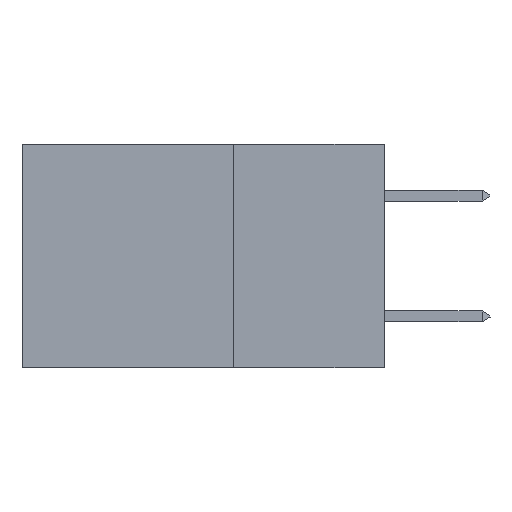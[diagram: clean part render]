
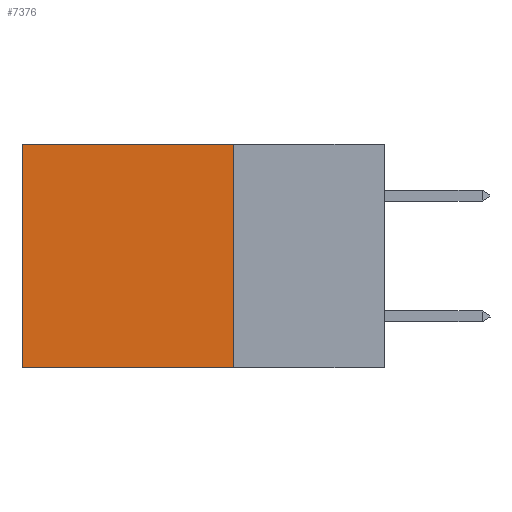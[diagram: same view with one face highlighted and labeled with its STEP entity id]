
A CAD part, left-side view. The second image highlights one B-rep face of the part: STEP entity #7376.
In plain terms, the highlighted planar face has unit normal (-1, 0, 0).
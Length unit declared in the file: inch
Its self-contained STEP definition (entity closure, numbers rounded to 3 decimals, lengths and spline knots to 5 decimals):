
#313 = CARTESIAN_POINT ( 'NONE',  ( 0.2875, 0.25, 0. ) ) ;
#563 = VECTOR ( 'NONE', #5628, 39.37008 ) ;
#585 = DIRECTION ( 'NONE',  ( 0., 0., -1. ) ) ;
#672 = CARTESIAN_POINT ( 'NONE',  ( 0.2875, 0.25, 0. ) ) ;
#883 = LINE ( 'NONE', #8996, #7415 ) ;
#1250 = DIRECTION ( 'NONE',  ( 0., 0., -1. ) ) ;
#1438 = FACE_OUTER_BOUND ( 'NONE', #3929, .T. ) ;
#1440 = DIRECTION ( 'NONE',  ( 1., 0., 0. ) ) ;
#1986 = LINE ( 'NONE', #8472, #563 ) ;
#2133 = ORIENTED_EDGE ( 'NONE', *, *, #6322, .F. ) ;
#2152 = CARTESIAN_POINT ( 'NONE',  ( 0.2875, 0.25, 0. ) ) ;
#2187 = PLANE ( 'NONE',  #6969 ) ;
#3240 = VERTEX_POINT ( 'NONE', #6380 ) ;
#3360 = VECTOR ( 'NONE', #7100, 39.37008 ) ;
#3609 = VERTEX_POINT ( 'NONE', #5166 ) ;
#3929 = EDGE_LOOP ( 'NONE', ( #6810, #2133, #7901, #4018 ) ) ;
#4018 = ORIENTED_EDGE ( 'NONE', *, *, #7542, .T. ) ;
#4304 = CARTESIAN_POINT ( 'NONE',  ( 0.2875, 0.25, 0. ) ) ;
#4471 = CARTESIAN_POINT ( 'NONE',  ( 0.2875, 0.6, 0. ) ) ;
#4871 = DIRECTION ( 'NONE',  ( 0., 0., -1. ) ) ;
#4913 = LINE ( 'NONE', #672, #5218 ) ;
#5166 = CARTESIAN_POINT ( 'NONE',  ( 0.2875, 0.6, -0.37 ) ) ;
#5218 = VECTOR ( 'NONE', #585, 39.37008 ) ;
#5628 = DIRECTION ( 'NONE',  ( 0., 1., 0. ) ) ;
#6322 = EDGE_CURVE ( 'NONE', #3240, #3609, #1986, .T. ) ;
#6380 = CARTESIAN_POINT ( 'NONE',  ( 0.2875, 0.25, -0.37 ) ) ;
#6810 = ORIENTED_EDGE ( 'NONE', *, *, #7013, .T. ) ;
#6969 = AXIS2_PLACEMENT_3D ( 'NONE', #2152, #1440, #4871 ) ;
#7013 = EDGE_CURVE ( 'NONE', #7145, #3609, #883, .T. ) ;
#7100 = DIRECTION ( 'NONE',  ( 0., 1., 0. ) ) ;
#7145 = VERTEX_POINT ( 'NONE', #4471 ) ;
#7210 = EDGE_CURVE ( 'NONE', #8713, #3240, #4913, .T. ) ;
#7376 = ADVANCED_FACE ( 'NONE', ( #1438 ), #2187, .F. ) ;
#7415 = VECTOR ( 'NONE', #1250, 39.37008 ) ;
#7542 = EDGE_CURVE ( 'NONE', #8713, #7145, #7859, .T. ) ;
#7859 = LINE ( 'NONE', #4304, #3360 ) ;
#7901 = ORIENTED_EDGE ( 'NONE', *, *, #7210, .F. ) ;
#8472 = CARTESIAN_POINT ( 'NONE',  ( 0.2875, 0.25, -0.37 ) ) ;
#8713 = VERTEX_POINT ( 'NONE', #313 ) ;
#8996 = CARTESIAN_POINT ( 'NONE',  ( 0.2875, 0.6, 0. ) ) ;
